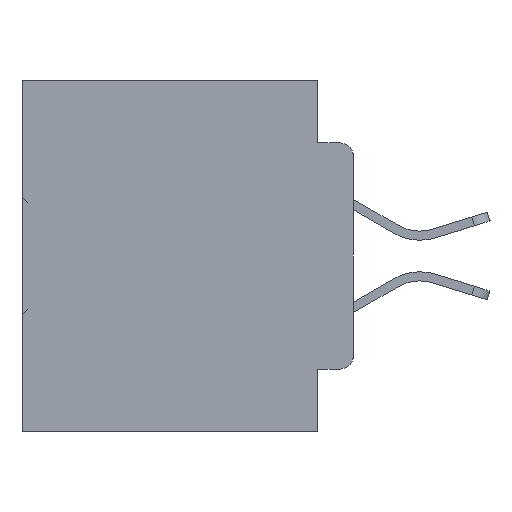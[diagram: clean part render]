
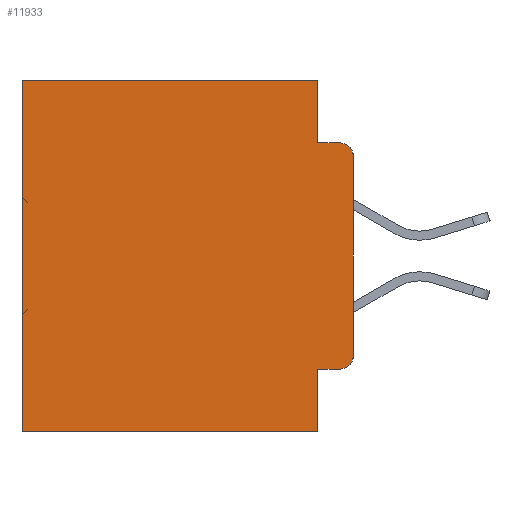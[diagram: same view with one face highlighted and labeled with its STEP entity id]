
A CAD part, left-side view. The second image highlights one B-rep face of the part: STEP entity #11933.
In plain terms, the highlighted planar face has unit normal (-1, 0, 0).
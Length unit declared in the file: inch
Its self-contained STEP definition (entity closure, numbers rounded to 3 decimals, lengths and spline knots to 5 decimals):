
#184 = EDGE_CURVE ( 'NONE', #26171, #22702, #11584, .T. ) ;
#1049 = DIRECTION ( 'NONE',  ( 0., 0., -1. ) ) ;
#1107 = DIRECTION ( 'NONE',  ( 0., 0., -1. ) ) ;
#2666 = AXIS2_PLACEMENT_3D ( 'NONE', #6861, #33146, #7056 ) ;
#3014 = CARTESIAN_POINT ( 'NONE',  ( 0.298, 0.051, -0.4115 ) ) ;
#3621 = LINE ( 'NONE', #14943, #30027 ) ;
#3745 = CARTESIAN_POINT ( 'NONE',  ( 0.298, 0., -0.3915 ) ) ;
#4349 = PLANE ( 'NONE',  #2666 ) ;
#5454 = AXIS2_PLACEMENT_3D ( 'NONE', #14532, #26243, #37956 ) ;
#5669 = DIRECTION ( 'NONE',  ( 0., 1., 0. ) ) ;
#6384 = CARTESIAN_POINT ( 'NONE',  ( 0.298, 0.051, -0.0885 ) ) ;
#6861 = CARTESIAN_POINT ( 'NONE',  ( 0.298, 0., 0. ) ) ;
#7009 = DIRECTION ( 'NONE',  ( 0., 1., 0. ) ) ;
#7056 = DIRECTION ( 'NONE',  ( 0., 0., -1. ) ) ;
#7296 = EDGE_CURVE ( 'NONE', #26171, #18583, #3621, .T. ) ;
#7421 = EDGE_CURVE ( 'NONE', #8171, #18583, #34315, .T. ) ;
#8003 = CARTESIAN_POINT ( 'NONE',  ( 0.298, 0.051, -0.4115 ) ) ;
#8171 = VERTEX_POINT ( 'NONE', #32162 ) ;
#8547 = CARTESIAN_POINT ( 'NONE',  ( 0.298, 0., 0. ) ) ;
#9105 = LINE ( 'NONE', #8547, #21184 ) ;
#10280 = CARTESIAN_POINT ( 'NONE',  ( 0.298, 0., -0.1085 ) ) ;
#10366 = ORIENTED_EDGE ( 'NONE', *, *, #14558, .F. ) ;
#10874 = LINE ( 'NONE', #8003, #27110 ) ;
#11332 = EDGE_CURVE ( 'NONE', #29553, #28206, #32255, .T. ) ;
#11584 = CIRCLE ( 'NONE', #5454, 0.02 ) ;
#11918 = LINE ( 'NONE', #23255, #32842 ) ;
#11933 = ADVANCED_FACE ( 'NONE', ( #21257 ), #4349, .F. ) ;
#12457 = EDGE_CURVE ( 'NONE', #21624, #27483, #30025, .T. ) ;
#12828 = DIRECTION ( 'NONE',  ( -1., 0., 0. ) ) ;
#13398 = CARTESIAN_POINT ( 'NONE',  ( 0.298, 0.02, -0.3915 ) ) ;
#13485 = ORIENTED_EDGE ( 'NONE', *, *, #7296, .F. ) ;
#13593 = ORIENTED_EDGE ( 'NONE', *, *, #18556, .F. ) ;
#13745 = DIRECTION ( 'NONE',  ( 0., -1., 0. ) ) ;
#14532 = CARTESIAN_POINT ( 'NONE',  ( 0.298, 0.02, -0.1085 ) ) ;
#14558 = EDGE_CURVE ( 'NONE', #28206, #22702, #18133, .T. ) ;
#14575 = DIRECTION ( 'NONE',  ( 0., 0., -1. ) ) ;
#14943 = CARTESIAN_POINT ( 'NONE',  ( 0.298, 0., 0. ) ) ;
#15418 = CARTESIAN_POINT ( 'NONE',  ( 0.298, 0., -0.5 ) ) ;
#16047 = VECTOR ( 'NONE', #1049, 39.37008 ) ;
#18133 = LINE ( 'NONE', #27350, #28311 ) ;
#18547 = CARTESIAN_POINT ( 'NONE',  ( 0.298, 0.473, -0.5 ) ) ;
#18556 = EDGE_CURVE ( 'NONE', #21868, #21624, #30243, .T. ) ;
#18583 = VERTEX_POINT ( 'NONE', #3745 ) ;
#18868 = ORIENTED_EDGE ( 'NONE', *, *, #11332, .F. ) ;
#19638 = CARTESIAN_POINT ( 'NONE',  ( 0.298, 0.473, 0. ) ) ;
#21184 = VECTOR ( 'NONE', #5669, 39.37008 ) ;
#21257 = FACE_OUTER_BOUND ( 'NONE', #27823, .T. ) ;
#21437 = ORIENTED_EDGE ( 'NONE', *, *, #22096, .T. ) ;
#21624 = VERTEX_POINT ( 'NONE', #31432 ) ;
#21868 = VERTEX_POINT ( 'NONE', #3014 ) ;
#22096 = EDGE_CURVE ( 'NONE', #21868, #8171, #10874, .T. ) ;
#22663 = AXIS2_PLACEMENT_3D ( 'NONE', #13398, #12828, #1107 ) ;
#22702 = VERTEX_POINT ( 'NONE', #29602 ) ;
#22738 = ORIENTED_EDGE ( 'NONE', *, *, #12457, .F. ) ;
#23255 = CARTESIAN_POINT ( 'NONE',  ( 0.298, 0.473, 0. ) ) ;
#23408 = DIRECTION ( 'NONE',  ( 0., 0., -1. ) ) ;
#23438 = DIRECTION ( 'NONE',  ( 0., 0., -1. ) ) ;
#25771 = EDGE_CURVE ( 'NONE', #28016, #27483, #11918, .T. ) ;
#26161 = ORIENTED_EDGE ( 'NONE', *, *, #7421, .T. ) ;
#26171 = VERTEX_POINT ( 'NONE', #10280 ) ;
#26243 = DIRECTION ( 'NONE',  ( -1., 0., 0. ) ) ;
#26959 = DIRECTION ( 'NONE',  ( 0., -1., 0. ) ) ;
#27110 = VECTOR ( 'NONE', #13745, 39.37008 ) ;
#27231 = VECTOR ( 'NONE', #14575, 39.37008 ) ;
#27350 = CARTESIAN_POINT ( 'NONE',  ( 0.298, 0.051, -0.0885 ) ) ;
#27483 = VERTEX_POINT ( 'NONE', #18547 ) ;
#27823 = EDGE_LOOP ( 'NONE', ( #13485, #36067, #10366, #18868, #36366, #30071, #22738, #13593, #21437, #26161 ) ) ;
#28016 = VERTEX_POINT ( 'NONE', #19638 ) ;
#28206 = VERTEX_POINT ( 'NONE', #6384 ) ;
#28311 = VECTOR ( 'NONE', #26959, 39.37008 ) ;
#29553 = VERTEX_POINT ( 'NONE', #29799 ) ;
#29602 = CARTESIAN_POINT ( 'NONE',  ( 0.298, 0.02, -0.0885 ) ) ;
#29799 = CARTESIAN_POINT ( 'NONE',  ( 0.298, 0.051, 0. ) ) ;
#30025 = LINE ( 'NONE', #15418, #34945 ) ;
#30027 = VECTOR ( 'NONE', #23408, 39.37008 ) ;
#30043 = CARTESIAN_POINT ( 'NONE',  ( 0.298, 0.051, 0. ) ) ;
#30071 = ORIENTED_EDGE ( 'NONE', *, *, #25771, .T. ) ;
#30243 = LINE ( 'NONE', #30043, #16047 ) ;
#31432 = CARTESIAN_POINT ( 'NONE',  ( 0.298, 0.051, -0.5 ) ) ;
#32162 = CARTESIAN_POINT ( 'NONE',  ( 0.298, 0.02, -0.4115 ) ) ;
#32255 = LINE ( 'NONE', #35699, #27231 ) ;
#32842 = VECTOR ( 'NONE', #23438, 39.37008 ) ;
#33118 = EDGE_CURVE ( 'NONE', #29553, #28016, #9105, .T. ) ;
#33146 = DIRECTION ( 'NONE',  ( 1., 0., 0. ) ) ;
#34315 = CIRCLE ( 'NONE', #22663, 0.02 ) ;
#34945 = VECTOR ( 'NONE', #7009, 39.37008 ) ;
#35699 = CARTESIAN_POINT ( 'NONE',  ( 0.298, 0.051, 0. ) ) ;
#36067 = ORIENTED_EDGE ( 'NONE', *, *, #184, .T. ) ;
#36366 = ORIENTED_EDGE ( 'NONE', *, *, #33118, .T. ) ;
#37956 = DIRECTION ( 'NONE',  ( 0., 0., -1. ) ) ;
